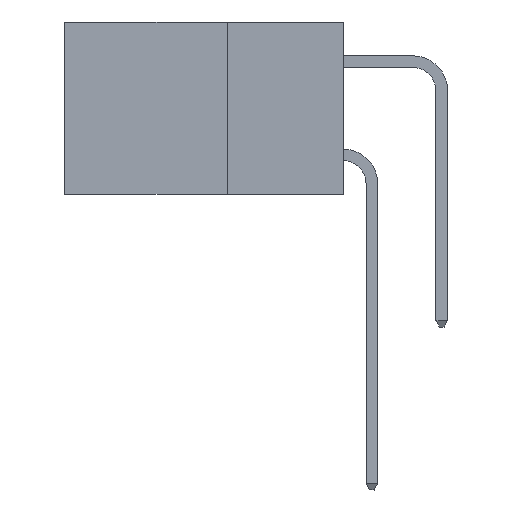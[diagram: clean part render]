
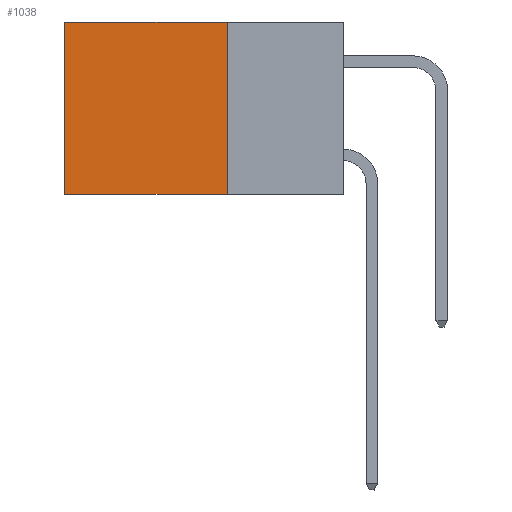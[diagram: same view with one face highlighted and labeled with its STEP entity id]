
A CAD part, left-side view. The second image highlights one B-rep face of the part: STEP entity #1038.
In plain terms, the highlighted planar face has unit normal (-1, 0, 0).
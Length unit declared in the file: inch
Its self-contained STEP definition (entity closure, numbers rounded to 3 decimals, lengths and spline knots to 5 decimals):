
#108 = LINE ( 'NONE', #18541, #19190 ) ;
#399 = VECTOR ( 'NONE', #773, 39.37008 ) ;
#773 = DIRECTION ( 'NONE',  ( 0., 1., 0. ) ) ;
#1038 = ADVANCED_FACE ( 'NONE', ( #17046 ), #10529, .F. ) ;
#1212 = LINE ( 'NONE', #17986, #8053 ) ;
#1257 = DIRECTION ( 'NONE',  ( 0., 0., -1. ) ) ;
#1699 = CARTESIAN_POINT ( 'NONE',  ( 0.2615, 0.6, -0.37 ) ) ;
#3035 = CARTESIAN_POINT ( 'NONE',  ( 0.2615, 0.25, 0. ) ) ;
#3325 = EDGE_CURVE ( 'NONE', #18126, #7820, #1212, .T. ) ;
#4433 = CARTESIAN_POINT ( 'NONE',  ( 0.2615, 0.25, -0.37 ) ) ;
#4827 = EDGE_CURVE ( 'NONE', #18126, #21500, #9787, .T. ) ;
#5459 = DIRECTION ( 'NONE',  ( 0., 0., -1. ) ) ;
#5509 = VERTEX_POINT ( 'NONE', #1699 ) ;
#7820 = VERTEX_POINT ( 'NONE', #12586 ) ;
#7953 = DIRECTION ( 'NONE',  ( 0., 1., 0. ) ) ;
#8053 = VECTOR ( 'NONE', #7953, 39.37008 ) ;
#8765 = CARTESIAN_POINT ( 'NONE',  ( 0.2615, 0.25, -0.37 ) ) ;
#9616 = ORIENTED_EDGE ( 'NONE', *, *, #3325, .T. ) ;
#9787 = LINE ( 'NONE', #19702, #11811 ) ;
#10470 = CARTESIAN_POINT ( 'NONE',  ( 0.2615, 0.25, -0.37 ) ) ;
#10529 = PLANE ( 'NONE',  #11160 ) ;
#10710 = ORIENTED_EDGE ( 'NONE', *, *, #4827, .F. ) ;
#11160 = AXIS2_PLACEMENT_3D ( 'NONE', #8765, #19013, #5459 ) ;
#11588 = EDGE_CURVE ( 'NONE', #21500, #5509, #16370, .T. ) ;
#11811 = VECTOR ( 'NONE', #21583, 39.37008 ) ;
#12586 = CARTESIAN_POINT ( 'NONE',  ( 0.2615, 0.6, 0. ) ) ;
#14429 = EDGE_LOOP ( 'NONE', ( #20778, #19733, #10710, #9616 ) ) ;
#16370 = LINE ( 'NONE', #4433, #399 ) ;
#17046 = FACE_OUTER_BOUND ( 'NONE', #14429, .T. ) ;
#17986 = CARTESIAN_POINT ( 'NONE',  ( 0.2615, 0.25, 0. ) ) ;
#18126 = VERTEX_POINT ( 'NONE', #3035 ) ;
#18541 = CARTESIAN_POINT ( 'NONE',  ( 0.2615, 0.6, -0.37 ) ) ;
#19013 = DIRECTION ( 'NONE',  ( 1., 0., 0. ) ) ;
#19190 = VECTOR ( 'NONE', #1257, 39.37008 ) ;
#19702 = CARTESIAN_POINT ( 'NONE',  ( 0.2615, 0.25, -0.37 ) ) ;
#19733 = ORIENTED_EDGE ( 'NONE', *, *, #11588, .F. ) ;
#20778 = ORIENTED_EDGE ( 'NONE', *, *, #21135, .T. ) ;
#21135 = EDGE_CURVE ( 'NONE', #7820, #5509, #108, .T. ) ;
#21500 = VERTEX_POINT ( 'NONE', #10470 ) ;
#21583 = DIRECTION ( 'NONE',  ( 0., 0., -1. ) ) ;
